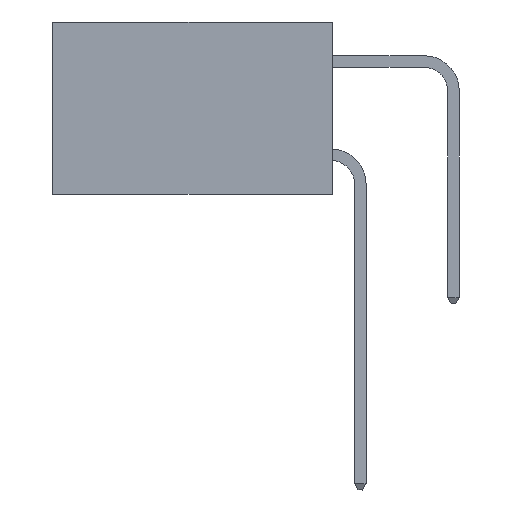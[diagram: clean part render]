
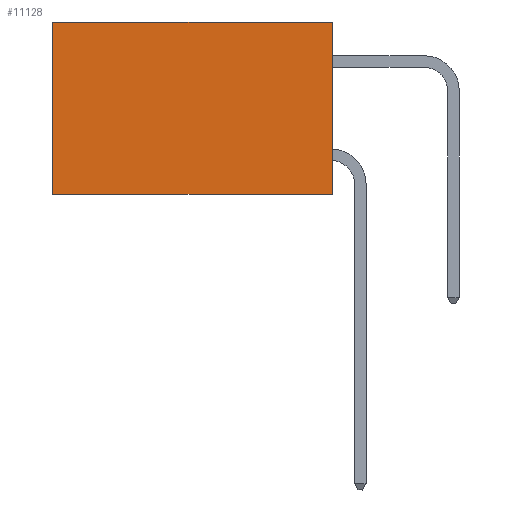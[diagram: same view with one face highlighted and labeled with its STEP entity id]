
A CAD part, left-side view. The second image highlights one B-rep face of the part: STEP entity #11128.
In plain terms, the highlighted planar face has unit normal (-1, 0, 0).
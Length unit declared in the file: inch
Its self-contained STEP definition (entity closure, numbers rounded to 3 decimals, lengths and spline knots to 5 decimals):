
#1451 = DIRECTION ( 'NONE',  ( 0., 0., -1. ) ) ;
#1635 = CARTESIAN_POINT ( 'NONE',  ( 0.298, 0., 0. ) ) ;
#2004 = DIRECTION ( 'NONE',  ( 0., 1., 0. ) ) ;
#2308 = DIRECTION ( 'NONE',  ( 0., 1., 0. ) ) ;
#3371 = CARTESIAN_POINT ( 'NONE',  ( 0.298, 0.6, -0.37 ) ) ;
#3743 = ORIENTED_EDGE ( 'NONE', *, *, #11232, .T. ) ;
#5933 = CARTESIAN_POINT ( 'NONE',  ( 0.298, 0., -0.37 ) ) ;
#5971 = VECTOR ( 'NONE', #2308, 39.37008 ) ;
#6032 = DIRECTION ( 'NONE',  ( 0., 0., -1. ) ) ;
#6353 = VECTOR ( 'NONE', #2004, 39.37008 ) ;
#6924 = EDGE_LOOP ( 'NONE', ( #3743, #14831, #15709, #23523 ) ) ;
#7969 = VERTEX_POINT ( 'NONE', #3371 ) ;
#8425 = AXIS2_PLACEMENT_3D ( 'NONE', #28779, #28365, #15030 ) ;
#8825 = LINE ( 'NONE', #15136, #29329 ) ;
#11128 = ADVANCED_FACE ( 'NONE', ( #28222 ), #25856, .F. ) ;
#11232 = EDGE_CURVE ( 'NONE', #21584, #7969, #8825, .T. ) ;
#12703 = LINE ( 'NONE', #16001, #6353 ) ;
#14831 = ORIENTED_EDGE ( 'NONE', *, *, #28947, .F. ) ;
#15030 = DIRECTION ( 'NONE',  ( 0., 0., -1. ) ) ;
#15136 = CARTESIAN_POINT ( 'NONE',  ( 0.298, 0.6, 0. ) ) ;
#15709 = ORIENTED_EDGE ( 'NONE', *, *, #26597, .F. ) ;
#16001 = CARTESIAN_POINT ( 'NONE',  ( 0.298, 0., 0. ) ) ;
#17581 = VERTEX_POINT ( 'NONE', #1635 ) ;
#18040 = CARTESIAN_POINT ( 'NONE',  ( 0.298, 0., 0. ) ) ;
#18300 = LINE ( 'NONE', #25984, #5971 ) ;
#18761 = CARTESIAN_POINT ( 'NONE',  ( 0.298, 0.6, 0. ) ) ;
#18803 = VECTOR ( 'NONE', #1451, 39.37008 ) ;
#21098 = VERTEX_POINT ( 'NONE', #5933 ) ;
#21584 = VERTEX_POINT ( 'NONE', #18761 ) ;
#21823 = LINE ( 'NONE', #18040, #18803 ) ;
#23523 = ORIENTED_EDGE ( 'NONE', *, *, #28803, .T. ) ;
#25856 = PLANE ( 'NONE',  #8425 ) ;
#25984 = CARTESIAN_POINT ( 'NONE',  ( 0.298, 0., -0.37 ) ) ;
#26597 = EDGE_CURVE ( 'NONE', #17581, #21098, #21823, .T. ) ;
#28222 = FACE_OUTER_BOUND ( 'NONE', #6924, .T. ) ;
#28365 = DIRECTION ( 'NONE',  ( 1., 0., 0. ) ) ;
#28779 = CARTESIAN_POINT ( 'NONE',  ( 0.298, 0., 0. ) ) ;
#28803 = EDGE_CURVE ( 'NONE', #17581, #21584, #12703, .T. ) ;
#28947 = EDGE_CURVE ( 'NONE', #21098, #7969, #18300, .T. ) ;
#29329 = VECTOR ( 'NONE', #6032, 39.37008 ) ;
